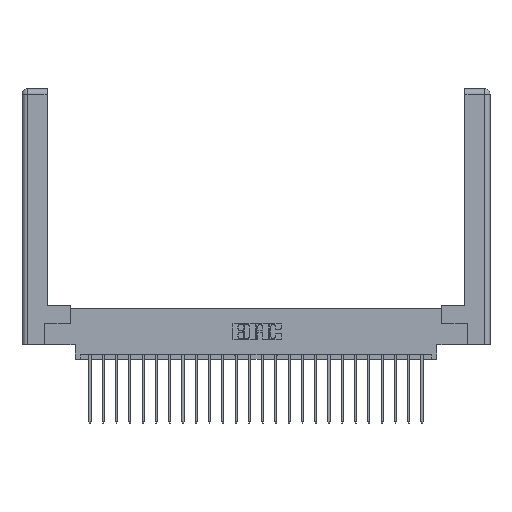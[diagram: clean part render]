
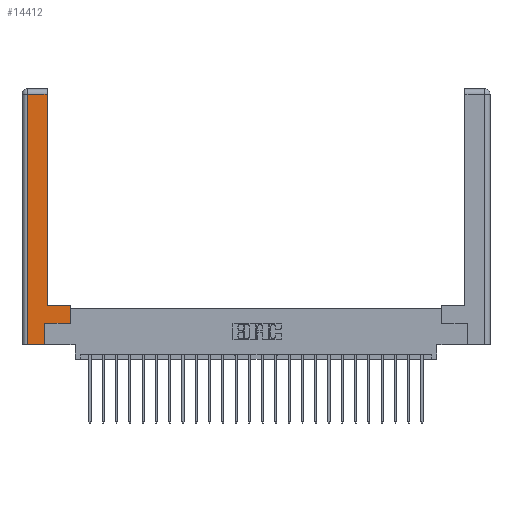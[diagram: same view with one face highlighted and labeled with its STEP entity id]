
A CAD part, top view. The second image highlights one B-rep face of the part: STEP entity #14412.
In plain terms, the highlighted planar face has unit normal (0, 0, 1).
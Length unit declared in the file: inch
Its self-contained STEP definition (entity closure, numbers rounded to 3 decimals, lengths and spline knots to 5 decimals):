
#628 = ORIENTED_EDGE ( 'NONE', *, *, #13860, .T. ) ;
#672 = EDGE_CURVE ( 'NONE', #13595, #20503, #11095, .T. ) ;
#926 = DIRECTION ( 'NONE',  ( 1., 0., 0. ) ) ;
#1260 = CARTESIAN_POINT ( 'NONE',  ( 0.295, 0.45, 0. ) ) ;
#1308 = DIRECTION ( 'NONE',  ( 0., 0., -1. ) ) ;
#1655 = EDGE_CURVE ( 'NONE', #20503, #5416, #12297, .T. ) ;
#1783 = ORIENTED_EDGE ( 'NONE', *, *, #9434, .T. ) ;
#2508 = CARTESIAN_POINT ( 'NONE',  ( 0.565, 0.245, 0. ) ) ;
#2572 = DIRECTION ( 'NONE',  ( -1., 0., 0. ) ) ;
#2699 = VERTEX_POINT ( 'NONE', #1260 ) ;
#2759 = ORIENTED_EDGE ( 'NONE', *, *, #22150, .T. ) ;
#3131 = CARTESIAN_POINT ( 'NONE',  ( 0., 0., 0. ) ) ;
#4016 = CARTESIAN_POINT ( 'NONE',  ( 0.565, 0.45, 0. ) ) ;
#4094 = DIRECTION ( 'NONE',  ( 0., 1., 0. ) ) ;
#4589 = VERTEX_POINT ( 'NONE', #18891 ) ;
#4781 = LINE ( 'NONE', #4016, #10237 ) ;
#5011 = PLANE ( 'NONE',  #11097 ) ;
#5416 = VERTEX_POINT ( 'NONE', #24103 ) ;
#6061 = VECTOR ( 'NONE', #18162, 39.37008 ) ;
#6108 = ORIENTED_EDGE ( 'NONE', *, *, #1655, .T. ) ;
#6235 = CARTESIAN_POINT ( 'NONE',  ( 0.295, 2.94, 0. ) ) ;
#7722 = CARTESIAN_POINT ( 'NONE',  ( 0.265, 0., 0. ) ) ;
#7807 = ORIENTED_EDGE ( 'NONE', *, *, #672, .T. ) ;
#7867 = ORIENTED_EDGE ( 'NONE', *, *, #9155, .T. ) ;
#8528 = CARTESIAN_POINT ( 'NONE',  ( 0.265, 0.245, 0. ) ) ;
#8593 = VERTEX_POINT ( 'NONE', #19967 ) ;
#8818 = LINE ( 'NONE', #8528, #6061 ) ;
#8924 = ORIENTED_EDGE ( 'NONE', *, *, #19257, .T. ) ;
#9155 = EDGE_CURVE ( 'NONE', #5416, #4589, #8818, .T. ) ;
#9434 = EDGE_CURVE ( 'NONE', #2699, #13202, #20880, .T. ) ;
#9511 = DIRECTION ( 'NONE',  ( 0., 1., 0. ) ) ;
#9937 = LINE ( 'NONE', #2508, #24433 ) ;
#10237 = VECTOR ( 'NONE', #4094, 39.37008 ) ;
#11095 = LINE ( 'NONE', #22385, #11707 ) ;
#11097 = AXIS2_PLACEMENT_3D ( 'NONE', #3131, #1308, #24239 ) ;
#11171 = CARTESIAN_POINT ( 'NONE',  ( 0.0615, 2.94, 0. ) ) ;
#11376 = EDGE_CURVE ( 'NONE', #13202, #13595, #23692, .T. ) ;
#11474 = ORIENTED_EDGE ( 'NONE', *, *, #11376, .T. ) ;
#11707 = VECTOR ( 'NONE', #12770, 39.37008 ) ;
#12297 = LINE ( 'NONE', #7722, #12896 ) ;
#12770 = DIRECTION ( 'NONE',  ( 0., -1., 0. ) ) ;
#12896 = VECTOR ( 'NONE', #21150, 39.37008 ) ;
#13202 = VERTEX_POINT ( 'NONE', #6235 ) ;
#13595 = VERTEX_POINT ( 'NONE', #11171 ) ;
#13860 = EDGE_CURVE ( 'NONE', #8593, #21454, #4781, .T. ) ;
#14351 = CARTESIAN_POINT ( 'NONE',  ( 0.565, 0.45, 0. ) ) ;
#14412 = ADVANCED_FACE ( 'NONE', ( #15677 ), #5011, .F. ) ;
#14526 = CARTESIAN_POINT ( 'NONE',  ( 0.295, 0.45, 0. ) ) ;
#15677 = FACE_OUTER_BOUND ( 'NONE', #23241, .T. ) ;
#16129 = VECTOR ( 'NONE', #19717, 39.37008 ) ;
#17701 = CARTESIAN_POINT ( 'NONE',  ( 0.0615, 2.94, 0. ) ) ;
#18162 = DIRECTION ( 'NONE',  ( 0., 1., 0. ) ) ;
#18497 = CARTESIAN_POINT ( 'NONE',  ( 0.0615, 0., 0. ) ) ;
#18891 = CARTESIAN_POINT ( 'NONE',  ( 0.265, 0.245, 0. ) ) ;
#19257 = EDGE_CURVE ( 'NONE', #4589, #8593, #9937, .T. ) ;
#19717 = DIRECTION ( 'NONE',  ( -1., 0., 0. ) ) ;
#19721 = LINE ( 'NONE', #14526, #24251 ) ;
#19967 = CARTESIAN_POINT ( 'NONE',  ( 0.565, 0.245, 0. ) ) ;
#20503 = VERTEX_POINT ( 'NONE', #18497 ) ;
#20880 = LINE ( 'NONE', #24980, #23323 ) ;
#21150 = DIRECTION ( 'NONE',  ( 1., 0., 0. ) ) ;
#21454 = VERTEX_POINT ( 'NONE', #14351 ) ;
#22150 = EDGE_CURVE ( 'NONE', #21454, #2699, #19721, .T. ) ;
#22385 = CARTESIAN_POINT ( 'NONE',  ( 0.0615, 0., 0. ) ) ;
#23241 = EDGE_LOOP ( 'NONE', ( #1783, #11474, #7807, #6108, #7867, #8924, #628, #2759 ) ) ;
#23323 = VECTOR ( 'NONE', #9511, 39.37008 ) ;
#23692 = LINE ( 'NONE', #17701, #16129 ) ;
#24103 = CARTESIAN_POINT ( 'NONE',  ( 0.265, 0., 0. ) ) ;
#24239 = DIRECTION ( 'NONE',  ( -1., 0., 0. ) ) ;
#24251 = VECTOR ( 'NONE', #2572, 39.37008 ) ;
#24433 = VECTOR ( 'NONE', #926, 39.37008 ) ;
#24980 = CARTESIAN_POINT ( 'NONE',  ( 0.295, 3., 0. ) ) ;
